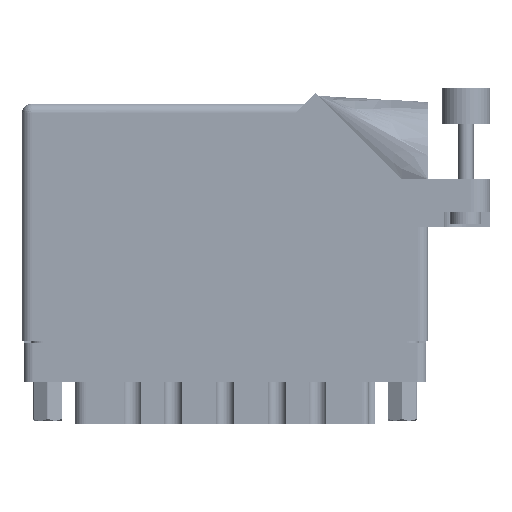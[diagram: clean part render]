
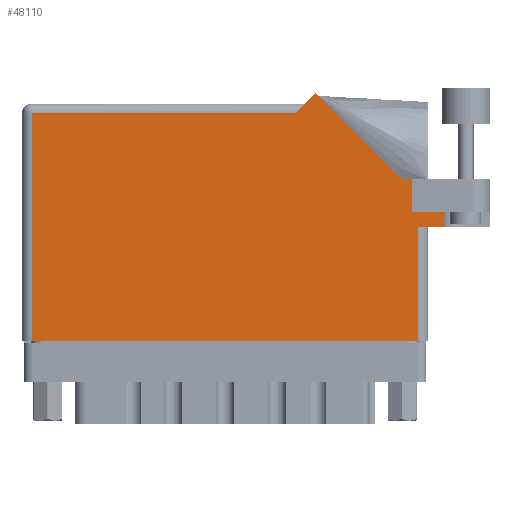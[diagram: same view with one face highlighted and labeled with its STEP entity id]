
A CAD part, front view. The second image highlights one B-rep face of the part: STEP entity #48110.
In plain terms, the highlighted face is planar.
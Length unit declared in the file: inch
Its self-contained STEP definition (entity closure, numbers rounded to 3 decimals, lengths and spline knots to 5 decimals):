
#183 = ORIENTED_EDGE ( 'NONE', *, *, #4986, .T. ) ;
#511 = VERTEX_POINT ( 'NONE', #13739 ) ;
#949 = DIRECTION ( 'NONE',  ( 0., 0., -1. ) ) ;
#1111 = DIRECTION ( 'NONE',  ( 0., 1., 0. ) ) ;
#1398 = ORIENTED_EDGE ( 'NONE', *, *, #61518, .T. ) ;
#2887 = DIRECTION ( 'NONE',  ( 1., 0., 0. ) ) ;
#3313 = LINE ( 'NONE', #26297, #59336 ) ;
#4737 = VECTOR ( 'NONE', #10038, 39.37008 ) ;
#4986 = EDGE_CURVE ( 'NONE', #45459, #60861, #60899, .T. ) ;
#5999 = CARTESIAN_POINT ( 'NONE',  ( 0., 1.53, 0. ) ) ;
#7229 = EDGE_CURVE ( 'NONE', #40232, #52822, #55345, .T. ) ;
#7822 = CARTESIAN_POINT ( 'NONE',  ( 0., 1.468, 0. ) ) ;
#8545 = CARTESIAN_POINT ( 'NONE',  ( 0.062, 1.468, 0. ) ) ;
#9240 = DIRECTION ( 'NONE',  ( 1., 0., 0. ) ) ;
#9505 = LINE ( 'NONE', #31847, #20108 ) ;
#10038 = DIRECTION ( 'NONE',  ( 0., -1., 0. ) ) ;
#12147 = VECTOR ( 'NONE', #41052, 39.37008 ) ;
#13739 = CARTESIAN_POINT ( 'NONE',  ( 2.55, 0., 0. ) ) ;
#14845 = EDGE_CURVE ( 'NONE', #29908, #45459, #25363, .T. ) ;
#15170 = CARTESIAN_POINT ( 'NONE',  ( 1.757, 1.468, 0. ) ) ;
#15976 = DIRECTION ( 'NONE',  ( 1., 0., 0. ) ) ;
#16337 = DIRECTION ( 'NONE',  ( -1., 0., 0. ) ) ;
#16468 = DIRECTION ( 'NONE',  ( -0.707, -0.707, 0. ) ) ;
#18709 = EDGE_CURVE ( 'NONE', #511, #27301, #25552, .T. ) ;
#18759 = CARTESIAN_POINT ( 'NONE',  ( 2.55, 0.737, 0. ) ) ;
#20108 = VECTOR ( 'NONE', #2887, 39.37008 ) ;
#20464 = CARTESIAN_POINT ( 'NONE',  ( 2.7135, 0.831, 0. ) ) ;
#20789 = DIRECTION ( 'NONE',  ( -0.707, 0.707, 0. ) ) ;
#21423 = ORIENTED_EDGE ( 'NONE', *, *, #34054, .T. ) ;
#24844 = EDGE_CURVE ( 'NONE', #27301, #52822, #33121, .T. ) ;
#25363 = LINE ( 'NONE', #30110, #45851 ) ;
#25552 = LINE ( 'NONE', #28473, #33900 ) ;
#25568 = VERTEX_POINT ( 'NONE', #38469 ) ;
#26297 = CARTESIAN_POINT ( 'NONE',  ( 3.012, 1.044, 0. ) ) ;
#26581 = CARTESIAN_POINT ( 'NONE',  ( 2.7135, 0.737, 0. ) ) ;
#27301 = VERTEX_POINT ( 'NONE', #18759 ) ;
#27902 = ORIENTED_EDGE ( 'NONE', *, *, #24844, .T. ) ;
#28156 = CARTESIAN_POINT ( 'NONE',  ( 1.88971, 1.60071, 0. ) ) ;
#28473 = CARTESIAN_POINT ( 'NONE',  ( 2.55, 0.737, 0. ) ) ;
#28653 = ORIENTED_EDGE ( 'NONE', *, *, #18709, .T. ) ;
#29908 = VERTEX_POINT ( 'NONE', #43895 ) ;
#30110 = CARTESIAN_POINT ( 'NONE',  ( 2.44642, 1.044, 0. ) ) ;
#30281 = ORIENTED_EDGE ( 'NONE', *, *, #14845, .T. ) ;
#30294 = DIRECTION ( 'NONE',  ( -1., 0., 0. ) ) ;
#30821 = AXIS2_PLACEMENT_3D ( 'NONE', #5999, #949, #30294 ) ;
#31193 = VERTEX_POINT ( 'NONE', #41584 ) ;
#31714 = EDGE_CURVE ( 'NONE', #60861, #52451, #42940, .T. ) ;
#31847 = CARTESIAN_POINT ( 'NONE',  ( 2.512, 0.831, 0. ) ) ;
#33121 = LINE ( 'NONE', #43141, #54298 ) ;
#33900 = VECTOR ( 'NONE', #39072, 39.37008 ) ;
#34054 = EDGE_CURVE ( 'NONE', #31193, #511, #48605, .T. ) ;
#34541 = CARTESIAN_POINT ( 'NONE',  ( 1.819, 1.53, 0. ) ) ;
#34993 = PLANE ( 'NONE',  #30821 ) ;
#38174 = EDGE_CURVE ( 'NONE', #48472, #40232, #9505, .T. ) ;
#38469 = CARTESIAN_POINT ( 'NONE',  ( 2.512, 1.044, 0. ) ) ;
#38610 = ORIENTED_EDGE ( 'NONE', *, *, #57565, .T. ) ;
#38855 = LINE ( 'NONE', #53434, #4737 ) ;
#39072 = DIRECTION ( 'NONE',  ( 0., 1., 0. ) ) ;
#40232 = VERTEX_POINT ( 'NONE', #20464 ) ;
#40434 = CARTESIAN_POINT ( 'NONE',  ( 2.512, 0.831, 0. ) ) ;
#41052 = DIRECTION ( 'NONE',  ( 0., -1., 0. ) ) ;
#41584 = CARTESIAN_POINT ( 'NONE',  ( 0.062, 0., 0. ) ) ;
#42940 = LINE ( 'NONE', #7822, #55031 ) ;
#43141 = CARTESIAN_POINT ( 'NONE',  ( 2.612, 0.737, 0. ) ) ;
#43895 = CARTESIAN_POINT ( 'NONE',  ( 2.44642, 1.044, 0. ) ) ;
#44831 = CARTESIAN_POINT ( 'NONE',  ( 0., 0., 0. ) ) ;
#45459 = VERTEX_POINT ( 'NONE', #28156 ) ;
#45765 = DIRECTION ( 'NONE',  ( -1., 0., 0. ) ) ;
#45851 = VECTOR ( 'NONE', #20789, 39.37008 ) ;
#46366 = ORIENTED_EDGE ( 'NONE', *, *, #62321, .T. ) ;
#48029 = VECTOR ( 'NONE', #16468, 39.37008 ) ;
#48110 = ADVANCED_FACE ( 'NONE', ( #48691 ), #34993, .F. ) ;
#48249 = LINE ( 'NONE', #40434, #55776 ) ;
#48472 = VERTEX_POINT ( 'NONE', #51682 ) ;
#48605 = LINE ( 'NONE', #44831, #51614 ) ;
#48691 = FACE_OUTER_BOUND ( 'NONE', #50003, .T. ) ;
#50003 = EDGE_LOOP ( 'NONE', ( #21423, #28653, #27902, #62725, #50072, #46366, #38610, #30281, #183, #52074, #1398 ) ) ;
#50072 = ORIENTED_EDGE ( 'NONE', *, *, #38174, .F. ) ;
#51614 = VECTOR ( 'NONE', #15976, 39.37008 ) ;
#51682 = CARTESIAN_POINT ( 'NONE',  ( 2.512, 0.831, 0. ) ) ;
#52074 = ORIENTED_EDGE ( 'NONE', *, *, #31714, .T. ) ;
#52451 = VERTEX_POINT ( 'NONE', #8545 ) ;
#52822 = VERTEX_POINT ( 'NONE', #26581 ) ;
#53434 = CARTESIAN_POINT ( 'NONE',  ( 0.062, 0., 0. ) ) ;
#54298 = VECTOR ( 'NONE', #9240, 39.37008 ) ;
#55031 = VECTOR ( 'NONE', #45765, 39.37008 ) ;
#55345 = LINE ( 'NONE', #60097, #12147 ) ;
#55776 = VECTOR ( 'NONE', #1111, 39.37008 ) ;
#57565 = EDGE_CURVE ( 'NONE', #25568, #29908, #3313, .T. ) ;
#59336 = VECTOR ( 'NONE', #16337, 39.37008 ) ;
#60097 = CARTESIAN_POINT ( 'NONE',  ( 2.7135, 1.16177, 0. ) ) ;
#60861 = VERTEX_POINT ( 'NONE', #15170 ) ;
#60899 = LINE ( 'NONE', #34541, #48029 ) ;
#61518 = EDGE_CURVE ( 'NONE', #52451, #31193, #38855, .T. ) ;
#62321 = EDGE_CURVE ( 'NONE', #48472, #25568, #48249, .T. ) ;
#62725 = ORIENTED_EDGE ( 'NONE', *, *, #7229, .F. ) ;
